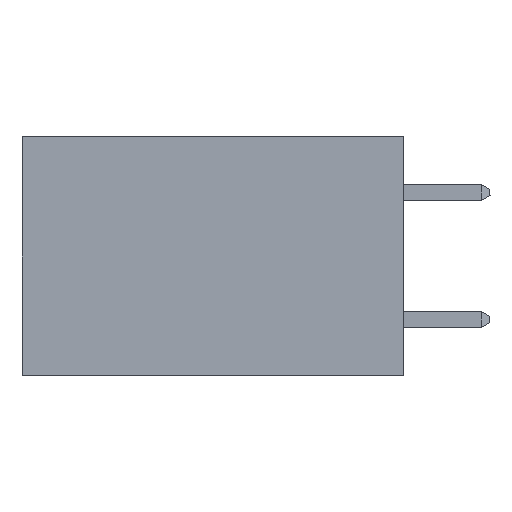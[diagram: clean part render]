
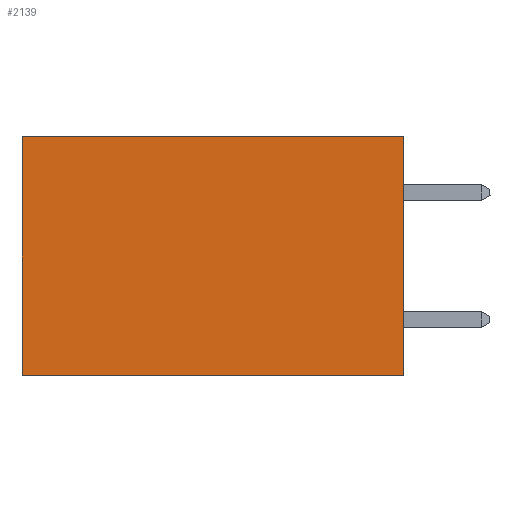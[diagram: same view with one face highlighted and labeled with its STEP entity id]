
A CAD part, left-side view. The second image highlights one B-rep face of the part: STEP entity #2139.
In plain terms, the highlighted planar face has unit normal (-1, 0, 0).
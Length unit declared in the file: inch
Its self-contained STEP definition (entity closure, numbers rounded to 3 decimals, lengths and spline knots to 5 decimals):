
#19 = LINE ( 'NONE', #5520, #4117 ) ;
#81 = VERTEX_POINT ( 'NONE', #3729 ) ;
#906 = VERTEX_POINT ( 'NONE', #3365 ) ;
#991 = FACE_OUTER_BOUND ( 'NONE', #6957, .T. ) ;
#1079 = LINE ( 'NONE', #5119, #5989 ) ;
#1317 = ORIENTED_EDGE ( 'NONE', *, *, #6584, .T. ) ;
#1337 = CARTESIAN_POINT ( 'NONE',  ( 0.2875, 0., -0.375 ) ) ;
#1361 = CARTESIAN_POINT ( 'NONE',  ( 0.2875, 0.6, 0. ) ) ;
#1950 = CARTESIAN_POINT ( 'NONE',  ( 0.2875, 0.6, -0.375 ) ) ;
#1968 = DIRECTION ( 'NONE',  ( 0., 1., 0. ) ) ;
#2139 = ADVANCED_FACE ( 'NONE', ( #991 ), #3228, .F. ) ;
#2163 = DIRECTION ( 'NONE',  ( 0., 0., -1. ) ) ;
#2848 = AXIS2_PLACEMENT_3D ( 'NONE', #7262, #6025, #2163 ) ;
#3162 = DIRECTION ( 'NONE',  ( 0., 0., -1. ) ) ;
#3228 = PLANE ( 'NONE',  #2848 ) ;
#3365 = CARTESIAN_POINT ( 'NONE',  ( 0.2875, 0., -0.375 ) ) ;
#3729 = CARTESIAN_POINT ( 'NONE',  ( 0.2875, 0., 0. ) ) ;
#4117 = VECTOR ( 'NONE', #4891, 39.37008 ) ;
#4373 = VERTEX_POINT ( 'NONE', #4760 ) ;
#4760 = CARTESIAN_POINT ( 'NONE',  ( 0.2875, 0.6, -0.375 ) ) ;
#4887 = VECTOR ( 'NONE', #1968, 39.37008 ) ;
#4891 = DIRECTION ( 'NONE',  ( 0., 1., 0. ) ) ;
#4903 = LINE ( 'NONE', #1950, #7137 ) ;
#5103 = DIRECTION ( 'NONE',  ( 0., 0., -1. ) ) ;
#5119 = CARTESIAN_POINT ( 'NONE',  ( 0.2875, 0., -0.375 ) ) ;
#5520 = CARTESIAN_POINT ( 'NONE',  ( 0.2875, 0., 0. ) ) ;
#5767 = VERTEX_POINT ( 'NONE', #1361 ) ;
#5989 = VECTOR ( 'NONE', #3162, 39.37008 ) ;
#6025 = DIRECTION ( 'NONE',  ( 1., 0., 0. ) ) ;
#6265 = ORIENTED_EDGE ( 'NONE', *, *, #7299, .T. ) ;
#6584 = EDGE_CURVE ( 'NONE', #5767, #4373, #4903, .T. ) ;
#6590 = LINE ( 'NONE', #1337, #4887 ) ;
#6957 = EDGE_LOOP ( 'NONE', ( #1317, #8238, #7706, #6265 ) ) ;
#7137 = VECTOR ( 'NONE', #5103, 39.37008 ) ;
#7262 = CARTESIAN_POINT ( 'NONE',  ( 0.2875, 0., -0.375 ) ) ;
#7299 = EDGE_CURVE ( 'NONE', #81, #5767, #19, .T. ) ;
#7706 = ORIENTED_EDGE ( 'NONE', *, *, #8151, .F. ) ;
#7740 = EDGE_CURVE ( 'NONE', #906, #4373, #6590, .T. ) ;
#8151 = EDGE_CURVE ( 'NONE', #81, #906, #1079, .T. ) ;
#8238 = ORIENTED_EDGE ( 'NONE', *, *, #7740, .F. ) ;
